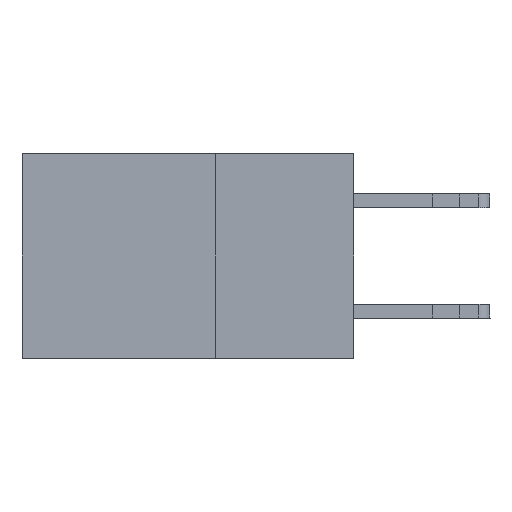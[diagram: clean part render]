
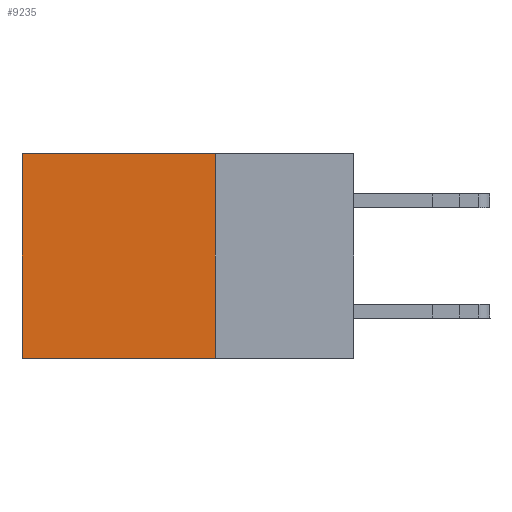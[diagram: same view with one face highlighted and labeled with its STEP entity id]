
A CAD part, left-side view. The second image highlights one B-rep face of the part: STEP entity #9235.
In plain terms, the highlighted planar face has unit normal (-1, 0, 0).
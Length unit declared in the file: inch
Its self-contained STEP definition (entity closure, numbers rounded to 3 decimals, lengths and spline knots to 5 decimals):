
#672 = CARTESIAN_POINT ( 'NONE',  ( 0.2875, 0.6, -0.37 ) ) ;
#1071 = VERTEX_POINT ( 'NONE', #672 ) ;
#1634 = CARTESIAN_POINT ( 'NONE',  ( 0.2875, 0.25, 0. ) ) ;
#1968 = CARTESIAN_POINT ( 'NONE',  ( 0.2875, 0.25, -0.37 ) ) ;
#2240 = VECTOR ( 'NONE', #24583, 39.37008 ) ;
#3025 = VECTOR ( 'NONE', #3585, 39.37008 ) ;
#3585 = DIRECTION ( 'NONE',  ( 0., 0., -1. ) ) ;
#3610 = CARTESIAN_POINT ( 'NONE',  ( 0.2875, 0.25, 0. ) ) ;
#3782 = DIRECTION ( 'NONE',  ( 1., 0., 0. ) ) ;
#4432 = VERTEX_POINT ( 'NONE', #25078 ) ;
#5830 = FACE_OUTER_BOUND ( 'NONE', #23391, .T. ) ;
#6030 = LINE ( 'NONE', #26956, #3025 ) ;
#6274 = ORIENTED_EDGE ( 'NONE', *, *, #6920, .F. ) ;
#6592 = LINE ( 'NONE', #3610, #23563 ) ;
#6920 = EDGE_CURVE ( 'NONE', #4432, #10033, #6030, .T. ) ;
#7547 = CARTESIAN_POINT ( 'NONE',  ( 0.2875, 0.25, -0.37 ) ) ;
#8068 = EDGE_CURVE ( 'NONE', #10033, #1071, #16250, .T. ) ;
#9235 = ADVANCED_FACE ( 'NONE', ( #5830 ), #12233, .F. ) ;
#9496 = VERTEX_POINT ( 'NONE', #26396 ) ;
#10033 = VERTEX_POINT ( 'NONE', #1968 ) ;
#11186 = ORIENTED_EDGE ( 'NONE', *, *, #25678, .T. ) ;
#12153 = DIRECTION ( 'NONE',  ( 0., 1., 0. ) ) ;
#12233 = PLANE ( 'NONE',  #16271 ) ;
#13217 = VECTOR ( 'NONE', #25323, 39.37008 ) ;
#13543 = LINE ( 'NONE', #16735, #13217 ) ;
#14956 = ORIENTED_EDGE ( 'NONE', *, *, #8068, .F. ) ;
#16250 = LINE ( 'NONE', #7547, #2240 ) ;
#16271 = AXIS2_PLACEMENT_3D ( 'NONE', #1634, #3782, #18682 ) ;
#16485 = ORIENTED_EDGE ( 'NONE', *, *, #25857, .T. ) ;
#16735 = CARTESIAN_POINT ( 'NONE',  ( 0.2875, 0.6, 0. ) ) ;
#18682 = DIRECTION ( 'NONE',  ( 0., 0., -1. ) ) ;
#23391 = EDGE_LOOP ( 'NONE', ( #16485, #14956, #6274, #11186 ) ) ;
#23563 = VECTOR ( 'NONE', #12153, 39.37008 ) ;
#24583 = DIRECTION ( 'NONE',  ( 0., 1., 0. ) ) ;
#25078 = CARTESIAN_POINT ( 'NONE',  ( 0.2875, 0.25, 0. ) ) ;
#25323 = DIRECTION ( 'NONE',  ( 0., 0., -1. ) ) ;
#25678 = EDGE_CURVE ( 'NONE', #4432, #9496, #6592, .T. ) ;
#25857 = EDGE_CURVE ( 'NONE', #9496, #1071, #13543, .T. ) ;
#26396 = CARTESIAN_POINT ( 'NONE',  ( 0.2875, 0.6, 0. ) ) ;
#26956 = CARTESIAN_POINT ( 'NONE',  ( 0.2875, 0.25, 0. ) ) ;
